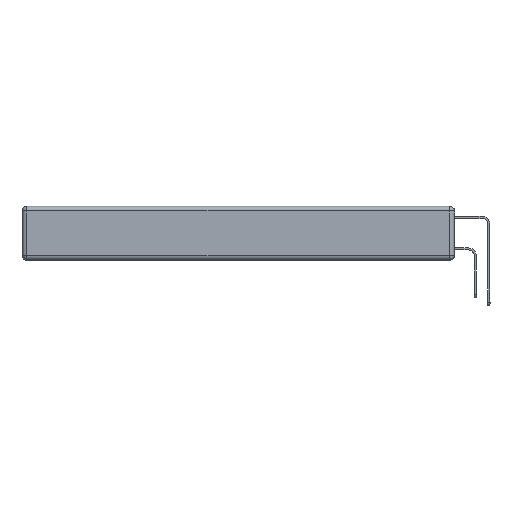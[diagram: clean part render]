
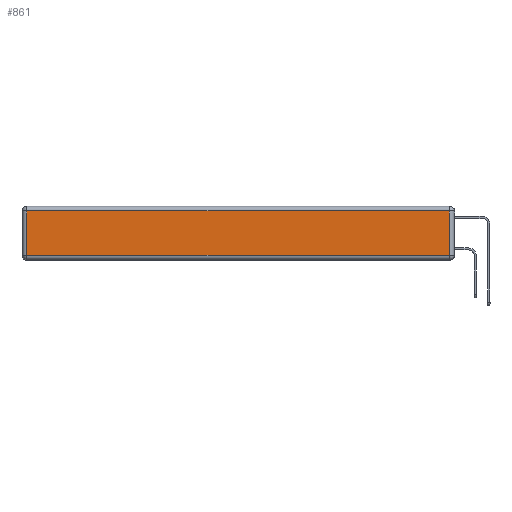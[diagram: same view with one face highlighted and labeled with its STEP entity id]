
A CAD part, left-side view. The second image highlights one B-rep face of the part: STEP entity #861.
In plain terms, the highlighted planar face has unit normal (-1, 0, 0).
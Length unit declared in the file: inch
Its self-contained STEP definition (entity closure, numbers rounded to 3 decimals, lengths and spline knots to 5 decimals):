
#861 = ADVANCED_FACE ( 'NONE', ( #5107 ), #9431, .T. ) ;
#978 = CARTESIAN_POINT ( 'NONE',  ( 0., 0.03, -0.343 ) ) ;
#1040 = CARTESIAN_POINT ( 'NONE',  ( 0., 0., -0.313 ) ) ;
#1059 = LINE ( 'NONE', #6515, #4396 ) ;
#1277 = LINE ( 'NONE', #13119, #5153 ) ;
#1714 = DIRECTION ( 'NONE',  ( 0., 0., 1. ) ) ;
#2059 = ORIENTED_EDGE ( 'NONE', *, *, #9408, .T. ) ;
#2144 = VERTEX_POINT ( 'NONE', #11300 ) ;
#2555 = CARTESIAN_POINT ( 'NONE',  ( 0., 0.03, -0.313 ) ) ;
#2775 = CARTESIAN_POINT ( 'NONE',  ( 0., 0., -0.343 ) ) ;
#3459 = DIRECTION ( 'NONE',  ( 0., -1., 0. ) ) ;
#3478 = DIRECTION ( 'NONE',  ( 0., 1., 0. ) ) ;
#4395 = DIRECTION ( 'NONE',  ( 0., 0., 1. ) ) ;
#4396 = VECTOR ( 'NONE', #13042, 39.37008 ) ;
#4660 = ORIENTED_EDGE ( 'NONE', *, *, #5678, .T. ) ;
#5107 = FACE_OUTER_BOUND ( 'NONE', #8030, .T. ) ;
#5153 = VECTOR ( 'NONE', #3478, 39.37008 ) ;
#5496 = VERTEX_POINT ( 'NONE', #6081 ) ;
#5678 = EDGE_CURVE ( 'NONE', #13256, #9488, #10766, .T. ) ;
#6081 = CARTESIAN_POINT ( 'NONE',  ( 0., 2.72, -0.03 ) ) ;
#6451 = EDGE_CURVE ( 'NONE', #5496, #13256, #1059, .T. ) ;
#6515 = CARTESIAN_POINT ( 'NONE',  ( 0., 2.72, -0.343 ) ) ;
#6977 = CARTESIAN_POINT ( 'NONE',  ( 0., 2.72, -0.313 ) ) ;
#8030 = EDGE_LOOP ( 'NONE', ( #4660, #12244, #2059, #10327 ) ) ;
#9367 = VECTOR ( 'NONE', #3459, 39.37008 ) ;
#9408 = EDGE_CURVE ( 'NONE', #2144, #5496, #1277, .T. ) ;
#9431 = PLANE ( 'NONE',  #9818 ) ;
#9488 = VERTEX_POINT ( 'NONE', #2555 ) ;
#9758 = EDGE_CURVE ( 'NONE', #9488, #2144, #10772, .T. ) ;
#9818 = AXIS2_PLACEMENT_3D ( 'NONE', #2775, #12417, #1714 ) ;
#10327 = ORIENTED_EDGE ( 'NONE', *, *, #6451, .T. ) ;
#10766 = LINE ( 'NONE', #1040, #9367 ) ;
#10772 = LINE ( 'NONE', #978, #11021 ) ;
#11021 = VECTOR ( 'NONE', #4395, 39.37008 ) ;
#11300 = CARTESIAN_POINT ( 'NONE',  ( 0., 0.03, -0.03 ) ) ;
#12244 = ORIENTED_EDGE ( 'NONE', *, *, #9758, .T. ) ;
#12417 = DIRECTION ( 'NONE',  ( -1., 0., 0. ) ) ;
#13042 = DIRECTION ( 'NONE',  ( 0., 0., -1. ) ) ;
#13119 = CARTESIAN_POINT ( 'NONE',  ( 0., 2.75, -0.03 ) ) ;
#13256 = VERTEX_POINT ( 'NONE', #6977 ) ;
